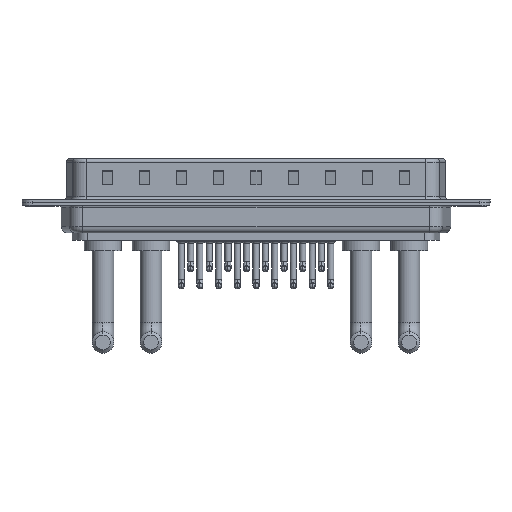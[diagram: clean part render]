
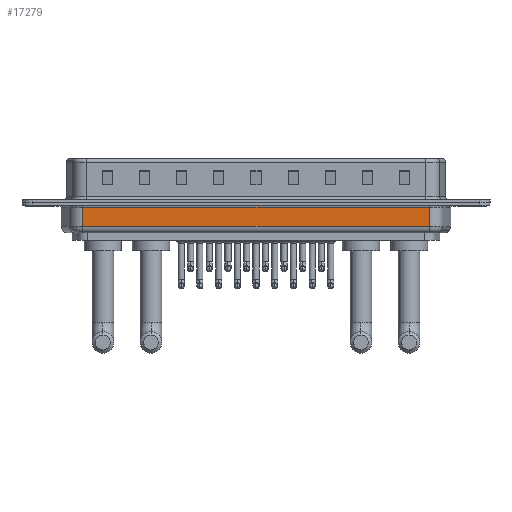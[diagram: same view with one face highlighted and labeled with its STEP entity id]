
A CAD part, front view. The second image highlights one B-rep face of the part: STEP entity #17279.
In plain terms, the highlighted planar face has unit normal (0, -1, 0).
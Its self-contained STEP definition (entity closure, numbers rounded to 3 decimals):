
#2544 = ORIENTED_EDGE ( 'NONE', *, *, #16427, .F. ) ;
#2935 = VECTOR ( 'NONE', #5300, 1000. ) ;
#3754 = FACE_OUTER_BOUND ( 'NONE', #4934, .T. ) ;
#4094 = DIRECTION ( 'NONE',  ( 0., 0., 1. ) ) ;
#4934 = EDGE_LOOP ( 'NONE', ( #2544, #11150, #19638, #17452 ) ) ;
#5071 = VECTOR ( 'NONE', #4094, 1000. ) ;
#5295 = EDGE_CURVE ( 'NONE', #6240, #24279, #16831, .T. ) ;
#5300 = DIRECTION ( 'NONE',  ( 0., 0., 1. ) ) ;
#5593 = CARTESIAN_POINT ( 'NONE',  ( 6.031, -5.35, -0.65 ) ) ;
#5652 = DIRECTION ( 'NONE',  ( 1., 0., 0. ) ) ;
#5757 = EDGE_CURVE ( 'NONE', #17812, #6240, #11468, .T. ) ;
#5792 = LINE ( 'NONE', #7823, #15939 ) ;
#6056 = CARTESIAN_POINT ( 'NONE',  ( 57.469, -5.35, -0.65 ) ) ;
#6240 = VERTEX_POINT ( 'NONE', #14986 ) ;
#6826 = CARTESIAN_POINT ( 'NONE',  ( 57.469, -5.35, -4.5 ) ) ;
#7669 = DIRECTION ( 'NONE',  ( -1., 0., 0. ) ) ;
#7823 = CARTESIAN_POINT ( 'NONE',  ( 6.031, -5.35, -0.65 ) ) ;
#8075 = DIRECTION ( 'NONE',  ( -1., 0., 0. ) ) ;
#9649 = LINE ( 'NONE', #11417, #5071 ) ;
#10050 = PLANE ( 'NONE',  #16409 ) ;
#11150 = ORIENTED_EDGE ( 'NONE', *, *, #5757, .T. ) ;
#11417 = CARTESIAN_POINT ( 'NONE',  ( 6.031, -5.35, -4.5 ) ) ;
#11468 = LINE ( 'NONE', #15526, #14279 ) ;
#14279 = VECTOR ( 'NONE', #5652, 1000. ) ;
#14986 = CARTESIAN_POINT ( 'NONE',  ( 57.469, -5.35, -3.5 ) ) ;
#15516 = DIRECTION ( 'NONE',  ( 0., 1., 0. ) ) ;
#15526 = CARTESIAN_POINT ( 'NONE',  ( 6.031, -5.35, -3.5 ) ) ;
#15581 = EDGE_CURVE ( 'NONE', #24279, #19904, #5792, .T. ) ;
#15939 = VECTOR ( 'NONE', #8075, 1000. ) ;
#16409 = AXIS2_PLACEMENT_3D ( 'NONE', #19175, #15516, #7669 ) ;
#16427 = EDGE_CURVE ( 'NONE', #17812, #19904, #9649, .T. ) ;
#16831 = LINE ( 'NONE', #6826, #2935 ) ;
#17279 = ADVANCED_FACE ( 'NONE', ( #3754 ), #10050, .F. ) ;
#17452 = ORIENTED_EDGE ( 'NONE', *, *, #15581, .T. ) ;
#17812 = VERTEX_POINT ( 'NONE', #20594 ) ;
#19175 = CARTESIAN_POINT ( 'NONE',  ( 6.031, -5.35, -4.5 ) ) ;
#19638 = ORIENTED_EDGE ( 'NONE', *, *, #5295, .T. ) ;
#19904 = VERTEX_POINT ( 'NONE', #5593 ) ;
#20594 = CARTESIAN_POINT ( 'NONE',  ( 6.031, -5.35, -3.5 ) ) ;
#24279 = VERTEX_POINT ( 'NONE', #6056 ) ;
